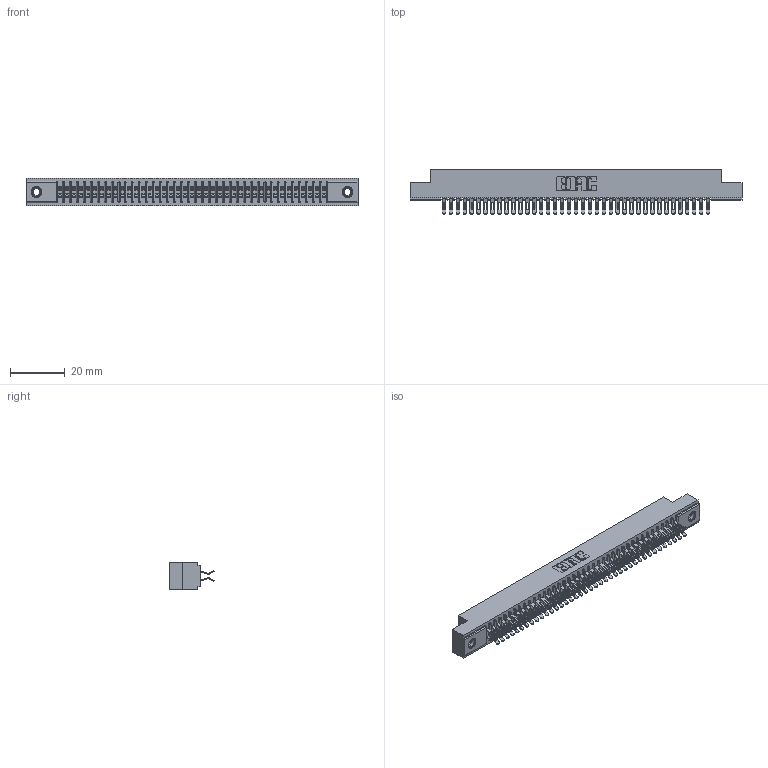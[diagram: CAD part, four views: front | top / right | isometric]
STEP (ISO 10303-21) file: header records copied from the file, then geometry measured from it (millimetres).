
FILE_DESCRIPTION (( 'STEP AP203' ), '1' );
FILE_NAME ('391-078-555-207.STEP', '2018-08-09T15:24:51', ( '' ), ( '' ), 'SwSTEP 2.0', 'SolidWorks 2016', '' );
FILE_SCHEMA (( 'CONFIG_CONTROL_DESIGN' ));
Length unit declared in the file: inch
Products named in the file (4): 391-078-555-207; 341 Part_.156 (3.96) Dia Mounting Holes; 341-292-001_341-292-155; 345-250-001_345-250-005-103
Assembly tree (81 placements, depth 2):
  391-078-555-207
    341 Part_.156 (3.96) Dia Mounting Holes
    341-292-001_341-292-155  x78
    345-250-001_345-250-005-103  x2
Bounding box: 121.28 x 16.31 x 10.16 mm (x, y, z)
Volume: 9039.3 mm3; surface area: 16622.9 mm2
Topology: 81 solids, 81 shells, 6260 faces, 18665 edges, 12146 vertices
Faces by surface type: plane 3376, cylinder 2712, sphere 80, torus 80, cone 12
Entity records: 49253 total; most frequent: CARTESIAN_POINT 8186, ORIENTED_EDGE 8118, DIRECTION 7947, EDGE_CURVE 4059, LINE 3257, VECTOR 3257, VERTEX_POINT 2568, AXIS2_PLACEMENT_3D 2345
